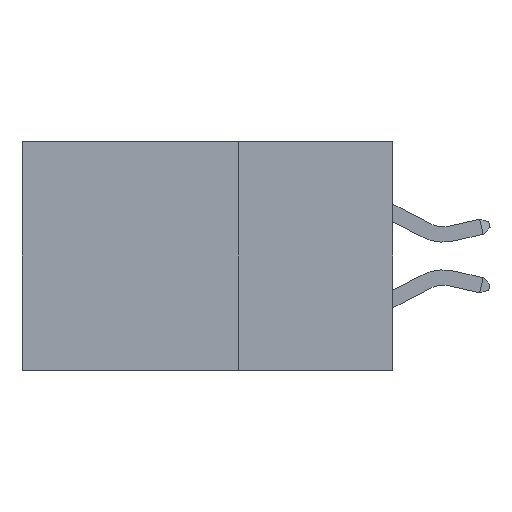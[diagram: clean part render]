
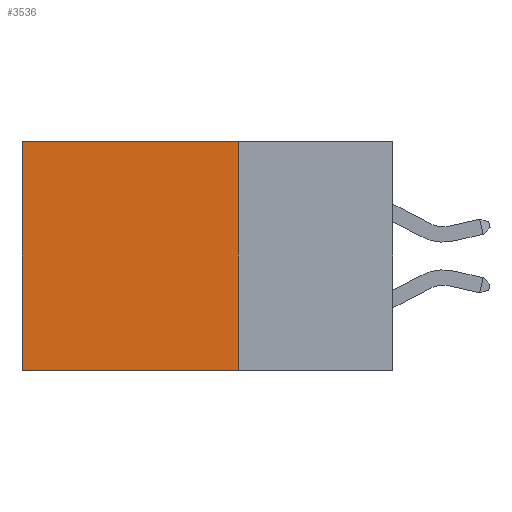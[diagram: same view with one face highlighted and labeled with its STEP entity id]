
A CAD part, left-side view. The second image highlights one B-rep face of the part: STEP entity #3536.
In plain terms, the highlighted planar face has unit normal (-1, 0, 0).
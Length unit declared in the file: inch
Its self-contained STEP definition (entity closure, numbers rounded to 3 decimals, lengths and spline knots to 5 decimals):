
#851 = VECTOR ( 'NONE', #23373, 39.37008 ) ;
#1481 = VECTOR ( 'NONE', #4054, 39.37008 ) ;
#1973 = ORIENTED_EDGE ( 'NONE', *, *, #18147, .F. ) ;
#2717 = CARTESIAN_POINT ( 'NONE',  ( 0.2875, 0.25, 0. ) ) ;
#3099 = CARTESIAN_POINT ( 'NONE',  ( 0.2875, 0.6, -0.37 ) ) ;
#3474 = LINE ( 'NONE', #9696, #5779 ) ;
#3536 = ADVANCED_FACE ( 'NONE', ( #15667 ), #9924, .F. ) ;
#3745 = LINE ( 'NONE', #20734, #6055 ) ;
#4054 = DIRECTION ( 'NONE',  ( 0., 1., 0. ) ) ;
#5779 = VECTOR ( 'NONE', #18852, 39.37008 ) ;
#6055 = VECTOR ( 'NONE', #22707, 39.37008 ) ;
#6152 = VERTEX_POINT ( 'NONE', #10125 ) ;
#9327 = LINE ( 'NONE', #12594, #851 ) ;
#9668 = VERTEX_POINT ( 'NONE', #21648 ) ;
#9696 = CARTESIAN_POINT ( 'NONE',  ( 0.2875, 0.25, 0. ) ) ;
#9924 = PLANE ( 'NONE',  #14141 ) ;
#10125 = CARTESIAN_POINT ( 'NONE',  ( 0.2875, 0.25, -0.37 ) ) ;
#10216 = EDGE_CURVE ( 'NONE', #9668, #22797, #9327, .T. ) ;
#11737 = DIRECTION ( 'NONE',  ( 0., 0., -1. ) ) ;
#11897 = CARTESIAN_POINT ( 'NONE',  ( 0.2875, 0.25, 0. ) ) ;
#12594 = CARTESIAN_POINT ( 'NONE',  ( 0.2875, 0.6, 0. ) ) ;
#14141 = AXIS2_PLACEMENT_3D ( 'NONE', #11897, #15487, #11737 ) ;
#14200 = LINE ( 'NONE', #14850, #1481 ) ;
#14850 = CARTESIAN_POINT ( 'NONE',  ( 0.2875, 0.25, -0.37 ) ) ;
#15487 = DIRECTION ( 'NONE',  ( 1., 0., 0. ) ) ;
#15667 = FACE_OUTER_BOUND ( 'NONE', #19453, .T. ) ;
#16060 = ORIENTED_EDGE ( 'NONE', *, *, #10216, .T. ) ;
#17943 = EDGE_CURVE ( 'NONE', #6152, #22797, #14200, .T. ) ;
#18108 = ORIENTED_EDGE ( 'NONE', *, *, #17943, .F. ) ;
#18147 = EDGE_CURVE ( 'NONE', #21065, #6152, #3474, .T. ) ;
#18852 = DIRECTION ( 'NONE',  ( 0., 0., -1. ) ) ;
#19453 = EDGE_LOOP ( 'NONE', ( #16060, #18108, #1973, #19740 ) ) ;
#19740 = ORIENTED_EDGE ( 'NONE', *, *, #22702, .T. ) ;
#20734 = CARTESIAN_POINT ( 'NONE',  ( 0.2875, 0.25, 0. ) ) ;
#21065 = VERTEX_POINT ( 'NONE', #2717 ) ;
#21648 = CARTESIAN_POINT ( 'NONE',  ( 0.2875, 0.6, 0. ) ) ;
#22702 = EDGE_CURVE ( 'NONE', #21065, #9668, #3745, .T. ) ;
#22707 = DIRECTION ( 'NONE',  ( 0., 1., 0. ) ) ;
#22797 = VERTEX_POINT ( 'NONE', #3099 ) ;
#23373 = DIRECTION ( 'NONE',  ( 0., 0., -1. ) ) ;
